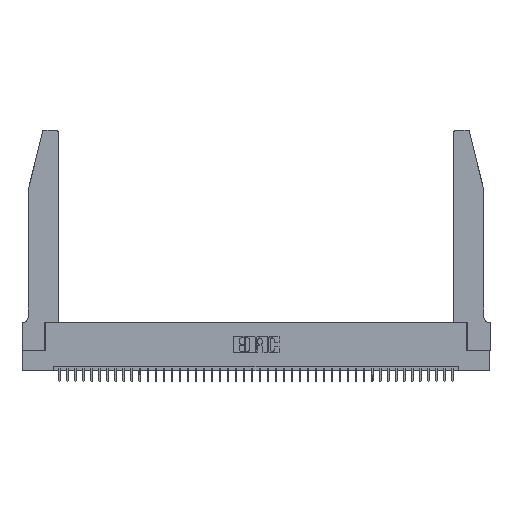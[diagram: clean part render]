
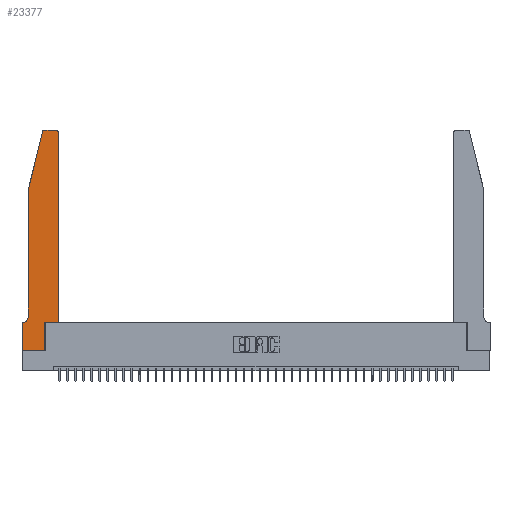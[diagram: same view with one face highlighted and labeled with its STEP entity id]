
A CAD part, top view. The second image highlights one B-rep face of the part: STEP entity #23377.
In plain terms, the highlighted planar face has unit normal (0, 0, 1).
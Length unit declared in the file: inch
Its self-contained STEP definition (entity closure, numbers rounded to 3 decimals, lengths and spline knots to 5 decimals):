
#43 = CARTESIAN_POINT ( 'NONE',  ( 0.0755, 2., 0.37 ) ) ;
#386 = VERTEX_POINT ( 'NONE', #27862 ) ;
#440 = DIRECTION ( 'NONE',  ( -0.239, -0.971, 0. ) ) ;
#845 = EDGE_CURVE ( 'NONE', #5173, #27402, #31488, .T. ) ;
#882 = DIRECTION ( 'NONE',  ( 1., 0., 0. ) ) ;
#1303 = PLANE ( 'NONE',  #2818 ) ;
#2309 = CARTESIAN_POINT ( 'NONE',  ( 0.2865, 0.35, 0.37 ) ) ;
#2818 = AXIS2_PLACEMENT_3D ( 'NONE', #40935, #24402, #27854 ) ;
#3271 = VECTOR ( 'NONE', #39389, 39.37008 ) ;
#3718 = VECTOR ( 'NONE', #34422, 39.37008 ) ;
#4263 = ORIENTED_EDGE ( 'NONE', *, *, #41651, .T. ) ;
#4546 = AXIS2_PLACEMENT_3D ( 'NONE', #23012, #19525, #36263 ) ;
#5024 = LINE ( 'NONE', #14839, #3718 ) ;
#5173 = VERTEX_POINT ( 'NONE', #20283 ) ;
#5257 = CARTESIAN_POINT ( 'NONE',  ( 0.0055, 0.35, 0.37 ) ) ;
#5357 = EDGE_CURVE ( 'NONE', #35204, #21902, #26144, .T. ) ;
#5730 = CARTESIAN_POINT ( 'NONE',  ( 0.4505, 0.35, 0.37 ) ) ;
#6500 = CARTESIAN_POINT ( 'NONE',  ( 0.4505, 0.35, 0.37 ) ) ;
#7366 = LINE ( 'NONE', #20667, #42611 ) ;
#8060 = CARTESIAN_POINT ( 'NONE',  ( 0.4205, 2.72, 0.37 ) ) ;
#8432 = DIRECTION ( 'NONE',  ( 0., -1., 0. ) ) ;
#8767 = CIRCLE ( 'NONE', #4546, 0.03 ) ;
#8933 = ORIENTED_EDGE ( 'NONE', *, *, #5357, .T. ) ;
#10295 = DIRECTION ( 'NONE',  ( 1., 0., 0. ) ) ;
#10456 = CIRCLE ( 'NONE', #15339, 0.07 ) ;
#10469 = EDGE_CURVE ( 'NONE', #16281, #5173, #7366, .T. ) ;
#10837 = ORIENTED_EDGE ( 'NONE', *, *, #30629, .T. ) ;
#11162 = CARTESIAN_POINT ( 'NONE',  ( 0.4205, 2.75, 0.37 ) ) ;
#11366 = CARTESIAN_POINT ( 'NONE',  ( 0.2865, 0., 0.37 ) ) ;
#11422 = CARTESIAN_POINT ( 'NONE',  ( 0.2605, 2.75, 0.37 ) ) ;
#11441 = VECTOR ( 'NONE', #24936, 39.37008 ) ;
#11499 = DIRECTION ( 'NONE',  ( -1., 0., 0. ) ) ;
#11541 = FACE_OUTER_BOUND ( 'NONE', #34273, .T. ) ;
#12879 = VERTEX_POINT ( 'NONE', #43 ) ;
#13959 = DIRECTION ( 'NONE',  ( 0., 0., 1. ) ) ;
#14362 = VERTEX_POINT ( 'NONE', #2309 ) ;
#14839 = CARTESIAN_POINT ( 'NONE',  ( 0.4505, 0.35, 0.37 ) ) ;
#15339 = AXIS2_PLACEMENT_3D ( 'NONE', #41584, #15667, #35475 ) ;
#15545 = DIRECTION ( 'NONE',  ( 0., 1., 0. ) ) ;
#15554 = EDGE_CURVE ( 'NONE', #39049, #25693, #8767, .T. ) ;
#15667 = DIRECTION ( 'NONE',  ( 0., 0., -1. ) ) ;
#15844 = ORIENTED_EDGE ( 'NONE', *, *, #15554, .T. ) ;
#16281 = VERTEX_POINT ( 'NONE', #5257 ) ;
#16593 = VECTOR ( 'NONE', #15545, 39.37008 ) ;
#18682 = CARTESIAN_POINT ( 'NONE',  ( 0., 0., 0.37 ) ) ;
#18714 = EDGE_CURVE ( 'NONE', #12879, #386, #32634, .T. ) ;
#19525 = DIRECTION ( 'NONE',  ( 0., 0., 1. ) ) ;
#20283 = CARTESIAN_POINT ( 'NONE',  ( 0., 0.35, 0.37 ) ) ;
#20667 = CARTESIAN_POINT ( 'NONE',  ( 0.0755, 0.35, 0.37 ) ) ;
#21740 = ORIENTED_EDGE ( 'NONE', *, *, #34981, .T. ) ;
#21902 = VERTEX_POINT ( 'NONE', #11162 ) ;
#22393 = CARTESIAN_POINT ( 'NONE',  ( 0.2865, 0.35, 0.37 ) ) ;
#23012 = CARTESIAN_POINT ( 'NONE',  ( 0.284, 2.72, 0.37 ) ) ;
#23377 = ADVANCED_FACE ( 'NONE', ( #11541 ), #1303, .T. ) ;
#23495 = EDGE_CURVE ( 'NONE', #386, #16281, #10456, .T. ) ;
#23980 = VECTOR ( 'NONE', #440, 39.37008 ) ;
#24402 = DIRECTION ( 'NONE',  ( 0., 0., 1. ) ) ;
#24936 = DIRECTION ( 'NONE',  ( -1., 0., 0. ) ) ;
#25693 = VERTEX_POINT ( 'NONE', #41040 ) ;
#26112 = CARTESIAN_POINT ( 'NONE',  ( 0.0755, 2., 0.37 ) ) ;
#26144 = CIRCLE ( 'NONE', #41419, 0.03 ) ;
#26910 = VECTOR ( 'NONE', #28910, 39.37008 ) ;
#27402 = VERTEX_POINT ( 'NONE', #42510 ) ;
#27814 = ORIENTED_EDGE ( 'NONE', *, *, #23495, .T. ) ;
#27854 = DIRECTION ( 'NONE',  ( 1., 0., 0. ) ) ;
#27862 = CARTESIAN_POINT ( 'NONE',  ( 0.0755, 0.42, 0.37 ) ) ;
#28265 = LINE ( 'NONE', #22393, #26910 ) ;
#28654 = VECTOR ( 'NONE', #8432, 39.37008 ) ;
#28910 = DIRECTION ( 'NONE',  ( 0., 1., 0. ) ) ;
#29138 = ORIENTED_EDGE ( 'NONE', *, *, #845, .T. ) ;
#30260 = CARTESIAN_POINT ( 'NONE',  ( 0.0755, 2., 0.37 ) ) ;
#30629 = EDGE_CURVE ( 'NONE', #14362, #32543, #5024, .T. ) ;
#31276 = ORIENTED_EDGE ( 'NONE', *, *, #10469, .T. ) ;
#31437 = EDGE_CURVE ( 'NONE', #21902, #39049, #41234, .T. ) ;
#31488 = LINE ( 'NONE', #18682, #28654 ) ;
#31811 = VERTEX_POINT ( 'NONE', #11366 ) ;
#32244 = EDGE_CURVE ( 'NONE', #25693, #12879, #33510, .T. ) ;
#32543 = VERTEX_POINT ( 'NONE', #6500 ) ;
#32594 = VECTOR ( 'NONE', #10295, 39.37008 ) ;
#32634 = LINE ( 'NONE', #26112, #3271 ) ;
#33377 = ORIENTED_EDGE ( 'NONE', *, *, #18714, .T. ) ;
#33510 = LINE ( 'NONE', #30260, #23980 ) ;
#34075 = CARTESIAN_POINT ( 'NONE',  ( 0.4505, 2.72, 0.37 ) ) ;
#34273 = EDGE_LOOP ( 'NONE', ( #36762, #15844, #34675, #33377, #27814, #31276, #29138, #4263, #21740, #10837, #42502, #8933 ) ) ;
#34422 = DIRECTION ( 'NONE',  ( 1., 0., 0. ) ) ;
#34675 = ORIENTED_EDGE ( 'NONE', *, *, #32244, .T. ) ;
#34981 = EDGE_CURVE ( 'NONE', #31811, #14362, #28265, .T. ) ;
#35204 = VERTEX_POINT ( 'NONE', #34075 ) ;
#35360 = LINE ( 'NONE', #5730, #16593 ) ;
#35475 = DIRECTION ( 'NONE',  ( -1., 0., 0. ) ) ;
#36009 = CARTESIAN_POINT ( 'NONE',  ( 0., 0., 0.37 ) ) ;
#36263 = DIRECTION ( 'NONE',  ( 1., 0., 0. ) ) ;
#36762 = ORIENTED_EDGE ( 'NONE', *, *, #31437, .T. ) ;
#36780 = CARTESIAN_POINT ( 'NONE',  ( 0.284, 2.75, 0.37 ) ) ;
#39049 = VERTEX_POINT ( 'NONE', #36780 ) ;
#39389 = DIRECTION ( 'NONE',  ( 0., -1., 0. ) ) ;
#39483 = LINE ( 'NONE', #36009, #32594 ) ;
#40935 = CARTESIAN_POINT ( 'NONE',  ( 0., 0.35, 0.37 ) ) ;
#41040 = CARTESIAN_POINT ( 'NONE',  ( 0.25487, 2.72718, 0.37 ) ) ;
#41234 = LINE ( 'NONE', #11422, #11441 ) ;
#41419 = AXIS2_PLACEMENT_3D ( 'NONE', #8060, #13959, #882 ) ;
#41584 = CARTESIAN_POINT ( 'NONE',  ( 0.0055, 0.42, 0.37 ) ) ;
#41594 = EDGE_CURVE ( 'NONE', #32543, #35204, #35360, .T. ) ;
#41651 = EDGE_CURVE ( 'NONE', #27402, #31811, #39483, .T. ) ;
#42502 = ORIENTED_EDGE ( 'NONE', *, *, #41594, .T. ) ;
#42510 = CARTESIAN_POINT ( 'NONE',  ( 0., 0., 0.37 ) ) ;
#42611 = VECTOR ( 'NONE', #11499, 39.37008 ) ;
